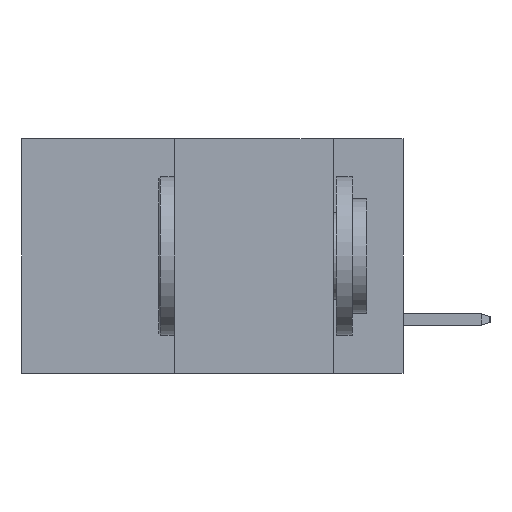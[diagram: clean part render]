
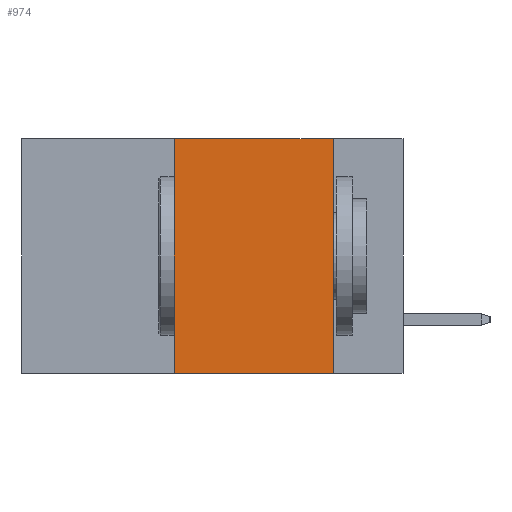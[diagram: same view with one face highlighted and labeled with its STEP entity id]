
A CAD part, left-side view. The second image highlights one B-rep face of the part: STEP entity #974.
In plain terms, the highlighted planar face has unit normal (-1, 0, 0).
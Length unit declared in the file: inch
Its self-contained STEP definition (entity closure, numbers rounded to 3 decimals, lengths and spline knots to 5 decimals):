
#64 = CARTESIAN_POINT ( 'NONE',  ( 0., 0.11, 0. ) ) ;
#110 = LINE ( 'NONE', #1824, #5453 ) ;
#814 = EDGE_CURVE ( 'NONE', #6362, #11851, #10128, .T. ) ;
#974 = ADVANCED_FACE ( 'NONE', ( #8748 ), #7762, .F. ) ;
#1006 = EDGE_CURVE ( 'NONE', #2406, #11851, #2261, .T. ) ;
#1577 = CARTESIAN_POINT ( 'NONE',  ( 0., 0.36, 0. ) ) ;
#1628 = VECTOR ( 'NONE', #9600, 39.37008 ) ;
#1824 = CARTESIAN_POINT ( 'NONE',  ( 0., 0.6, 0. ) ) ;
#2261 = LINE ( 'NONE', #4895, #1628 ) ;
#2406 = VERTEX_POINT ( 'NONE', #8707 ) ;
#2549 = CARTESIAN_POINT ( 'NONE',  ( 0., 0.11, 0. ) ) ;
#2685 = VERTEX_POINT ( 'NONE', #9487 ) ;
#2931 = DIRECTION ( 'NONE',  ( 1., 0., 0. ) ) ;
#3721 = DIRECTION ( 'NONE',  ( 0., -1., 0. ) ) ;
#4272 = DIRECTION ( 'NONE',  ( 0., 0., 1. ) ) ;
#4673 = ORIENTED_EDGE ( 'NONE', *, *, #6095, .F. ) ;
#4840 = EDGE_LOOP ( 'NONE', ( #9779, #4673, #9902, #10062 ) ) ;
#4895 = CARTESIAN_POINT ( 'NONE',  ( 0., 0.6, -0.37 ) ) ;
#5453 = VECTOR ( 'NONE', #3721, 39.37008 ) ;
#5582 = VECTOR ( 'NONE', #11883, 39.37008 ) ;
#5926 = AXIS2_PLACEMENT_3D ( 'NONE', #8559, #2931, #11509 ) ;
#6095 = EDGE_CURVE ( 'NONE', #2685, #6362, #110, .T. ) ;
#6362 = VERTEX_POINT ( 'NONE', #2549 ) ;
#7762 = PLANE ( 'NONE',  #5926 ) ;
#8559 = CARTESIAN_POINT ( 'NONE',  ( 0., 0.6, 0. ) ) ;
#8707 = CARTESIAN_POINT ( 'NONE',  ( 0., 0.36, -0.37 ) ) ;
#8748 = FACE_OUTER_BOUND ( 'NONE', #4840, .T. ) ;
#8933 = CARTESIAN_POINT ( 'NONE',  ( 0., 0.11, -0.37 ) ) ;
#9487 = CARTESIAN_POINT ( 'NONE',  ( 0., 0.36, 0. ) ) ;
#9600 = DIRECTION ( 'NONE',  ( 0., -1., 0. ) ) ;
#9779 = ORIENTED_EDGE ( 'NONE', *, *, #814, .F. ) ;
#9902 = ORIENTED_EDGE ( 'NONE', *, *, #11882, .F. ) ;
#10033 = LINE ( 'NONE', #1577, #11423 ) ;
#10062 = ORIENTED_EDGE ( 'NONE', *, *, #1006, .T. ) ;
#10128 = LINE ( 'NONE', #64, #5582 ) ;
#11423 = VECTOR ( 'NONE', #4272, 39.37008 ) ;
#11509 = DIRECTION ( 'NONE',  ( 0., 0., -1. ) ) ;
#11851 = VERTEX_POINT ( 'NONE', #8933 ) ;
#11882 = EDGE_CURVE ( 'NONE', #2406, #2685, #10033, .T. ) ;
#11883 = DIRECTION ( 'NONE',  ( 0., 0., -1. ) ) ;
